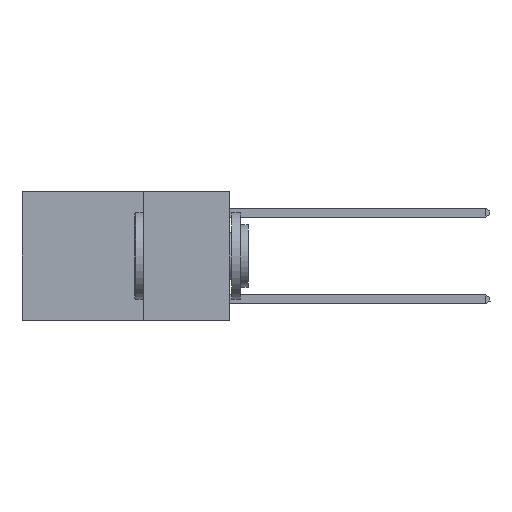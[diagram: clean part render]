
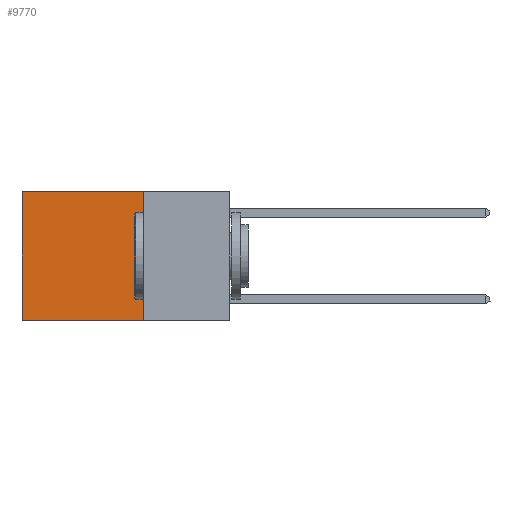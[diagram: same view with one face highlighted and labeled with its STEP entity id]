
A CAD part, left-side view. The second image highlights one B-rep face of the part: STEP entity #9770.
In plain terms, the highlighted planar face has unit normal (-1, 0, 0).
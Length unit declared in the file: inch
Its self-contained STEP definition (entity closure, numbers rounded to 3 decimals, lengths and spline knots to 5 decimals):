
#1 = PLANE ( 'NONE',  #2096 ) ;
#147 = CARTESIAN_POINT ( 'NONE',  ( 0.2625, 0.25, 0. ) ) ;
#604 = EDGE_CURVE ( 'NONE', #5223, #8361, #11030, .T. ) ;
#1431 = DIRECTION ( 'NONE',  ( 0., 0., -1. ) ) ;
#1534 = ORIENTED_EDGE ( 'NONE', *, *, #8955, .F. ) ;
#2096 = AXIS2_PLACEMENT_3D ( 'NONE', #10300, #5714, #3839 ) ;
#2415 = EDGE_LOOP ( 'NONE', ( #11929, #3826, #1534, #3098 ) ) ;
#2429 = CARTESIAN_POINT ( 'NONE',  ( 0.2625, 0.25, -0.37 ) ) ;
#2441 = VERTEX_POINT ( 'NONE', #2958 ) ;
#2559 = LINE ( 'NONE', #9968, #8540 ) ;
#2717 = VECTOR ( 'NONE', #10953, 39.37008 ) ;
#2958 = CARTESIAN_POINT ( 'NONE',  ( 0.2625, 0.25, 0. ) ) ;
#3098 = ORIENTED_EDGE ( 'NONE', *, *, #10644, .T. ) ;
#3449 = VERTEX_POINT ( 'NONE', #6885 ) ;
#3826 = ORIENTED_EDGE ( 'NONE', *, *, #604, .F. ) ;
#3839 = DIRECTION ( 'NONE',  ( 0., 0., -1. ) ) ;
#4453 = LINE ( 'NONE', #10996, #2717 ) ;
#4559 = FACE_OUTER_BOUND ( 'NONE', #2415, .T. ) ;
#5223 = VERTEX_POINT ( 'NONE', #9337 ) ;
#5334 = LINE ( 'NONE', #147, #11198 ) ;
#5714 = DIRECTION ( 'NONE',  ( 1., 0., 0. ) ) ;
#6678 = VECTOR ( 'NONE', #9039, 39.37008 ) ;
#6885 = CARTESIAN_POINT ( 'NONE',  ( 0.2625, 0.6, 0. ) ) ;
#8361 = VERTEX_POINT ( 'NONE', #9781 ) ;
#8467 = EDGE_CURVE ( 'NONE', #3449, #8361, #4453, .T. ) ;
#8540 = VECTOR ( 'NONE', #1431, 39.37008 ) ;
#8955 = EDGE_CURVE ( 'NONE', #2441, #5223, #2559, .T. ) ;
#9039 = DIRECTION ( 'NONE',  ( 0., 1., 0. ) ) ;
#9337 = CARTESIAN_POINT ( 'NONE',  ( 0.2625, 0.25, -0.37 ) ) ;
#9393 = DIRECTION ( 'NONE',  ( 0., 1., 0. ) ) ;
#9770 = ADVANCED_FACE ( 'NONE', ( #4559 ), #1, .F. ) ;
#9781 = CARTESIAN_POINT ( 'NONE',  ( 0.2625, 0.6, -0.37 ) ) ;
#9968 = CARTESIAN_POINT ( 'NONE',  ( 0.2625, 0.25, 0. ) ) ;
#10300 = CARTESIAN_POINT ( 'NONE',  ( 0.2625, 0.25, 0. ) ) ;
#10644 = EDGE_CURVE ( 'NONE', #2441, #3449, #5334, .T. ) ;
#10953 = DIRECTION ( 'NONE',  ( 0., 0., -1. ) ) ;
#10996 = CARTESIAN_POINT ( 'NONE',  ( 0.2625, 0.6, 0. ) ) ;
#11030 = LINE ( 'NONE', #2429, #6678 ) ;
#11198 = VECTOR ( 'NONE', #9393, 39.37008 ) ;
#11929 = ORIENTED_EDGE ( 'NONE', *, *, #8467, .T. ) ;
